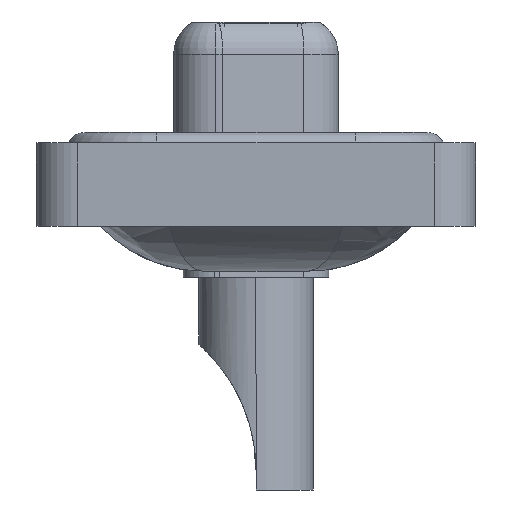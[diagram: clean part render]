
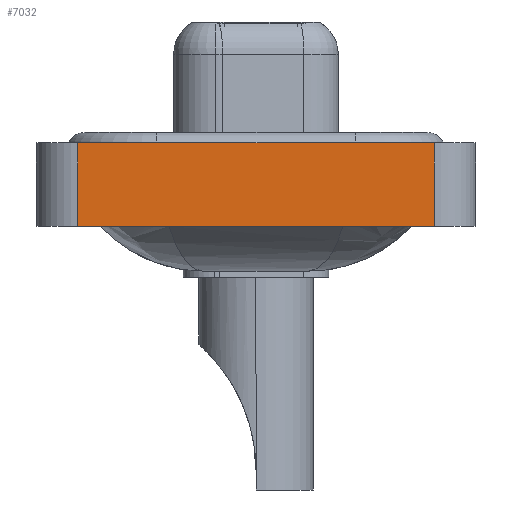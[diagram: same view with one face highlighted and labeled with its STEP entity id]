
A CAD part, left-side view. The second image highlights one B-rep face of the part: STEP entity #7032.
In plain terms, the highlighted planar face has unit normal (-1, 0, 0).
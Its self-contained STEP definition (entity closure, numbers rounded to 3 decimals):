
#77 = VECTOR ( 'NONE', #13297, 1000. ) ;
#162 = CARTESIAN_POINT ( 'NONE',  ( -7.35, -8.55, -3.6 ) ) ;
#362 = PLANE ( 'NONE',  #4546 ) ;
#617 = EDGE_CURVE ( 'NONE', #7052, #7141, #17191, .T. ) ;
#1006 = EDGE_CURVE ( 'NONE', #7141, #5655, #16121, .T. ) ;
#2200 = CARTESIAN_POINT ( 'NONE',  ( -7.35, -8.55, 0.4 ) ) ;
#3250 = FACE_OUTER_BOUND ( 'NONE', #14192, .T. ) ;
#3348 = CARTESIAN_POINT ( 'NONE',  ( -7.35, 8.55, -3.6 ) ) ;
#3623 = EDGE_CURVE ( 'NONE', #7052, #4568, #19042, .T. ) ;
#4546 = AXIS2_PLACEMENT_3D ( 'NONE', #11878, #6820, #16523 ) ;
#4568 = VERTEX_POINT ( 'NONE', #11848 ) ;
#5237 = DIRECTION ( 'NONE',  ( 0., -1., 0. ) ) ;
#5655 = VERTEX_POINT ( 'NONE', #2200 ) ;
#6180 = CARTESIAN_POINT ( 'NONE',  ( -7.35, -8.55, 0.4 ) ) ;
#6820 = DIRECTION ( 'NONE',  ( -1., 0., 0. ) ) ;
#6988 = EDGE_CURVE ( 'NONE', #4568, #5655, #12119, .T. ) ;
#7032 = ADVANCED_FACE ( 'NONE', ( #3250 ), #362, .T. ) ;
#7040 = CARTESIAN_POINT ( 'NONE',  ( -7.35, -8.55, -3.6 ) ) ;
#7052 = VERTEX_POINT ( 'NONE', #3348 ) ;
#7141 = VERTEX_POINT ( 'NONE', #7040 ) ;
#7789 = ORIENTED_EDGE ( 'NONE', *, *, #617, .T. ) ;
#11203 = ORIENTED_EDGE ( 'NONE', *, *, #1006, .T. ) ;
#11745 = VECTOR ( 'NONE', #5237, 1000. ) ;
#11848 = CARTESIAN_POINT ( 'NONE',  ( -7.35, 8.55, 0.4 ) ) ;
#11878 = CARTESIAN_POINT ( 'NONE',  ( -7.35, -8.55, -3.6 ) ) ;
#11925 = ORIENTED_EDGE ( 'NONE', *, *, #6988, .F. ) ;
#12119 = LINE ( 'NONE', #6180, #17650 ) ;
#13297 = DIRECTION ( 'NONE',  ( 0., 0., 1. ) ) ;
#14192 = EDGE_LOOP ( 'NONE', ( #11203, #11925, #19207, #7789 ) ) ;
#14483 = VECTOR ( 'NONE', #20449, 1000. ) ;
#16121 = LINE ( 'NONE', #162, #77 ) ;
#16523 = DIRECTION ( 'NONE',  ( 0., 0., 1. ) ) ;
#17119 = CARTESIAN_POINT ( 'NONE',  ( -7.35, 8.55, -3.6 ) ) ;
#17191 = LINE ( 'NONE', #20423, #11745 ) ;
#17650 = VECTOR ( 'NONE', #19318, 1000. ) ;
#19042 = LINE ( 'NONE', #17119, #14483 ) ;
#19207 = ORIENTED_EDGE ( 'NONE', *, *, #3623, .F. ) ;
#19318 = DIRECTION ( 'NONE',  ( 0., -1., 0. ) ) ;
#20423 = CARTESIAN_POINT ( 'NONE',  ( -7.35, -8.55, -3.6 ) ) ;
#20449 = DIRECTION ( 'NONE',  ( 0., 0., 1. ) ) ;
